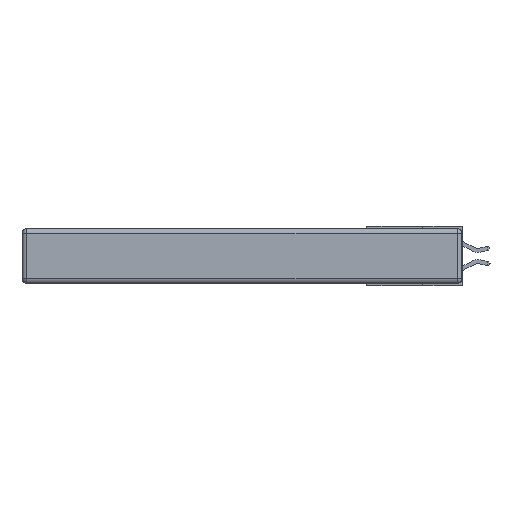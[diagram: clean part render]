
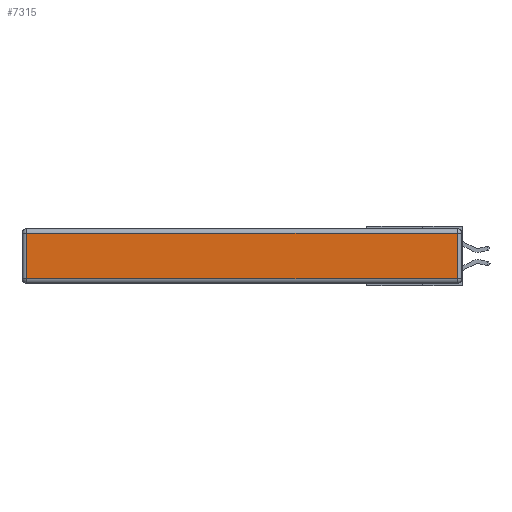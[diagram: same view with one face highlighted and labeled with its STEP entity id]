
A CAD part, left-side view. The second image highlights one B-rep face of the part: STEP entity #7315.
In plain terms, the highlighted planar face has unit normal (-1, 0, 0).
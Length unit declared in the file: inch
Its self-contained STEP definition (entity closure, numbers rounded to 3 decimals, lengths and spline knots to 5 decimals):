
#1859 = CARTESIAN_POINT ( 'NONE',  ( 0., 0., -0.343 ) ) ;
#3498 = VECTOR ( 'NONE', #20505, 39.37008 ) ;
#4273 = CARTESIAN_POINT ( 'NONE',  ( 0., 2.72, -0.313 ) ) ;
#4298 = VERTEX_POINT ( 'NONE', #4273 ) ;
#5116 = FACE_OUTER_BOUND ( 'NONE', #12482, .T. ) ;
#5264 = VERTEX_POINT ( 'NONE', #20272 ) ;
#5470 = ORIENTED_EDGE ( 'NONE', *, *, #25122, .T. ) ;
#5581 = VERTEX_POINT ( 'NONE', #15303 ) ;
#5631 = VECTOR ( 'NONE', #9692, 39.37008 ) ;
#6649 = ORIENTED_EDGE ( 'NONE', *, *, #25423, .T. ) ;
#7097 = CARTESIAN_POINT ( 'NONE',  ( 0., 2.72, -0.343 ) ) ;
#7315 = ADVANCED_FACE ( 'NONE', ( #5116 ), #25004, .T. ) ;
#7390 = CARTESIAN_POINT ( 'NONE',  ( 0., 0.03, -0.343 ) ) ;
#8586 = ORIENTED_EDGE ( 'NONE', *, *, #22344, .T. ) ;
#9692 = DIRECTION ( 'NONE',  ( 0., 1., 0. ) ) ;
#9967 = CARTESIAN_POINT ( 'NONE',  ( 0., 2.75, -0.03 ) ) ;
#11373 = VECTOR ( 'NONE', #13601, 39.37008 ) ;
#12328 = LINE ( 'NONE', #15277, #19883 ) ;
#12403 = DIRECTION ( 'NONE',  ( 0., 0., 1. ) ) ;
#12482 = EDGE_LOOP ( 'NONE', ( #6649, #5470, #8586, #21295 ) ) ;
#12848 = AXIS2_PLACEMENT_3D ( 'NONE', #1859, #20765, #12403 ) ;
#13601 = DIRECTION ( 'NONE',  ( 0., 0., -1. ) ) ;
#14665 = LINE ( 'NONE', #7390, #3498 ) ;
#14757 = VERTEX_POINT ( 'NONE', #24874 ) ;
#15277 = CARTESIAN_POINT ( 'NONE',  ( 0., 0., -0.313 ) ) ;
#15303 = CARTESIAN_POINT ( 'NONE',  ( 0., 0.03, -0.313 ) ) ;
#19127 = DIRECTION ( 'NONE',  ( 0., -1., 0. ) ) ;
#19883 = VECTOR ( 'NONE', #19127, 39.37008 ) ;
#20272 = CARTESIAN_POINT ( 'NONE',  ( 0., 0.03, -0.03 ) ) ;
#20505 = DIRECTION ( 'NONE',  ( 0., 0., 1. ) ) ;
#20765 = DIRECTION ( 'NONE',  ( -1., 0., 0. ) ) ;
#21295 = ORIENTED_EDGE ( 'NONE', *, *, #25655, .T. ) ;
#22344 = EDGE_CURVE ( 'NONE', #5264, #14757, #26309, .T. ) ;
#24159 = LINE ( 'NONE', #7097, #11373 ) ;
#24874 = CARTESIAN_POINT ( 'NONE',  ( 0., 2.72, -0.03 ) ) ;
#25004 = PLANE ( 'NONE',  #12848 ) ;
#25122 = EDGE_CURVE ( 'NONE', #5581, #5264, #14665, .T. ) ;
#25423 = EDGE_CURVE ( 'NONE', #4298, #5581, #12328, .T. ) ;
#25655 = EDGE_CURVE ( 'NONE', #14757, #4298, #24159, .T. ) ;
#26309 = LINE ( 'NONE', #9967, #5631 ) ;
